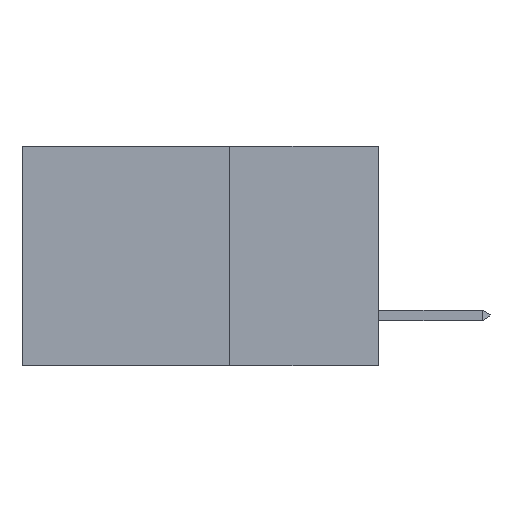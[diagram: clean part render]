
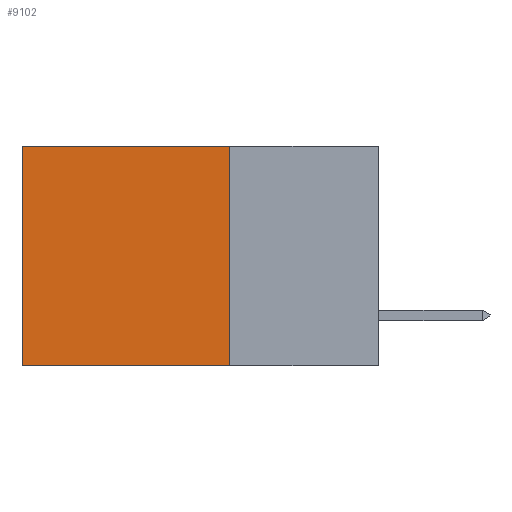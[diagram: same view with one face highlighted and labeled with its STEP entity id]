
A CAD part, left-side view. The second image highlights one B-rep face of the part: STEP entity #9102.
In plain terms, the highlighted planar face has unit normal (-1, 0, 0).
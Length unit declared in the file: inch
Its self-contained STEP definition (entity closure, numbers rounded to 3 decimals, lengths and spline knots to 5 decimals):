
#36 = VECTOR ( 'NONE', #7168, 39.37008 ) ;
#545 = VERTEX_POINT ( 'NONE', #1628 ) ;
#546 = DIRECTION ( 'NONE',  ( 0., 1., 0. ) ) ;
#683 = CARTESIAN_POINT ( 'NONE',  ( 0.298, 0.25, 0. ) ) ;
#742 = LINE ( 'NONE', #683, #1679 ) ;
#1405 = EDGE_CURVE ( 'NONE', #545, #5817, #742, .T. ) ;
#1628 = CARTESIAN_POINT ( 'NONE',  ( 0.298, 0.25, 0. ) ) ;
#1679 = VECTOR ( 'NONE', #8382, 39.37008 ) ;
#1760 = AXIS2_PLACEMENT_3D ( 'NONE', #1770, #2630, #1876 ) ;
#1770 = CARTESIAN_POINT ( 'NONE',  ( 0.298, 0.25, 0. ) ) ;
#1876 = DIRECTION ( 'NONE',  ( 0., 0., -1. ) ) ;
#2239 = CARTESIAN_POINT ( 'NONE',  ( 0.298, 0.6, 0. ) ) ;
#2630 = DIRECTION ( 'NONE',  ( 1., 0., 0. ) ) ;
#3631 = CARTESIAN_POINT ( 'NONE',  ( 0.298, 0.25, -0.37 ) ) ;
#3749 = CARTESIAN_POINT ( 'NONE',  ( 0.298, 0.6, -0.37 ) ) ;
#4367 = VERTEX_POINT ( 'NONE', #3631 ) ;
#4636 = ORIENTED_EDGE ( 'NONE', *, *, #1405, .T. ) ;
#4711 = VERTEX_POINT ( 'NONE', #3749 ) ;
#5189 = EDGE_CURVE ( 'NONE', #5817, #4711, #5609, .T. ) ;
#5298 = ORIENTED_EDGE ( 'NONE', *, *, #5189, .T. ) ;
#5609 = LINE ( 'NONE', #7082, #10015 ) ;
#5817 = VERTEX_POINT ( 'NONE', #2239 ) ;
#5942 = VECTOR ( 'NONE', #546, 39.37008 ) ;
#6180 = ORIENTED_EDGE ( 'NONE', *, *, #8393, .F. ) ;
#7082 = CARTESIAN_POINT ( 'NONE',  ( 0.298, 0.6, 0. ) ) ;
#7110 = FACE_OUTER_BOUND ( 'NONE', #10847, .T. ) ;
#7168 = DIRECTION ( 'NONE',  ( 0., 0., -1. ) ) ;
#7198 = DIRECTION ( 'NONE',  ( 0., 0., -1. ) ) ;
#7358 = ORIENTED_EDGE ( 'NONE', *, *, #8882, .F. ) ;
#7362 = CARTESIAN_POINT ( 'NONE',  ( 0.298, 0.25, -0.37 ) ) ;
#7400 = LINE ( 'NONE', #10566, #36 ) ;
#7693 = PLANE ( 'NONE',  #1760 ) ;
#7900 = LINE ( 'NONE', #7362, #5942 ) ;
#8382 = DIRECTION ( 'NONE',  ( 0., 1., 0. ) ) ;
#8393 = EDGE_CURVE ( 'NONE', #545, #4367, #7400, .T. ) ;
#8882 = EDGE_CURVE ( 'NONE', #4367, #4711, #7900, .T. ) ;
#9102 = ADVANCED_FACE ( 'NONE', ( #7110 ), #7693, .F. ) ;
#10015 = VECTOR ( 'NONE', #7198, 39.37008 ) ;
#10566 = CARTESIAN_POINT ( 'NONE',  ( 0.298, 0.25, 0. ) ) ;
#10847 = EDGE_LOOP ( 'NONE', ( #5298, #7358, #6180, #4636 ) ) ;
